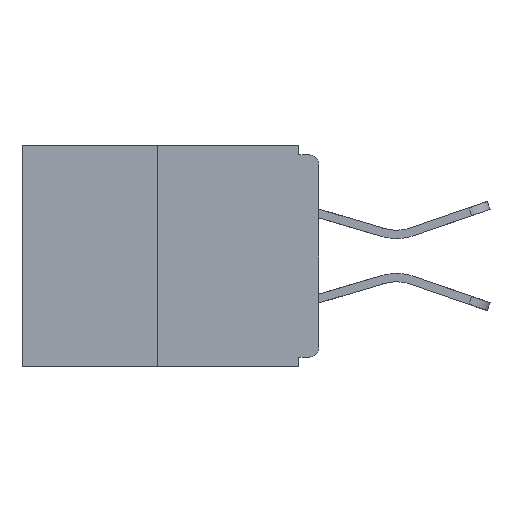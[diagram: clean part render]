
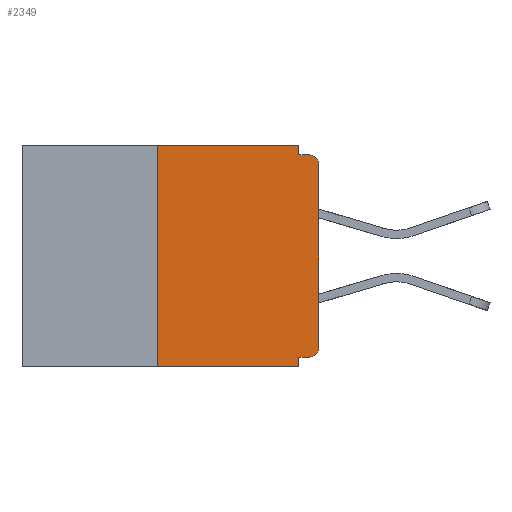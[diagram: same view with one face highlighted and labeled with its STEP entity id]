
A CAD part, left-side view. The second image highlights one B-rep face of the part: STEP entity #2349.
In plain terms, the highlighted planar face has unit normal (-1, 0, 0).
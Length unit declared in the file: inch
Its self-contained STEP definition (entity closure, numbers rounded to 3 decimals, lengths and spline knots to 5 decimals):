
#137 = VERTEX_POINT ( 'NONE', #14953 ) ;
#634 = CARTESIAN_POINT ( 'NONE',  ( 0., 0.015, -0.328 ) ) ;
#707 = DIRECTION ( 'NONE',  ( 0., -1., 0. ) ) ;
#886 = DIRECTION ( 'NONE',  ( 0., 0., -1. ) ) ;
#1024 = DIRECTION ( 'NONE',  ( 0., 0., -1. ) ) ;
#1085 = VERTEX_POINT ( 'NONE', #8054 ) ;
#1168 = PLANE ( 'NONE',  #6863 ) ;
#1349 = CARTESIAN_POINT ( 'NONE',  ( 0., 0.46, 0. ) ) ;
#1537 = AXIS2_PLACEMENT_3D ( 'NONE', #3720, #2639, #1024 ) ;
#1743 = EDGE_CURVE ( 'NONE', #15521, #137, #3775, .T. ) ;
#2099 = EDGE_CURVE ( 'NONE', #8170, #8888, #12645, .T. ) ;
#2170 = VECTOR ( 'NONE', #886, 39.37008 ) ;
#2233 = CARTESIAN_POINT ( 'NONE',  ( 0., 0., -0.015 ) ) ;
#2260 = DIRECTION ( 'NONE',  ( 0., -1., 0. ) ) ;
#2349 = ADVANCED_FACE ( 'NONE', ( #10765 ), #1168, .F. ) ;
#2639 = DIRECTION ( 'NONE',  ( -1., 0., 0. ) ) ;
#3092 = LINE ( 'NONE', #6608, #7737 ) ;
#3720 = CARTESIAN_POINT ( 'NONE',  ( 0., 0.015, -0.313 ) ) ;
#3775 = CIRCLE ( 'NONE', #1537, 0.015 ) ;
#4321 = CARTESIAN_POINT ( 'NONE',  ( 0., 0.031, 0. ) ) ;
#4432 = EDGE_CURVE ( 'NONE', #6960, #8888, #12793, .T. ) ;
#5322 = LINE ( 'NONE', #8947, #5982 ) ;
#5438 = DIRECTION ( 'NONE',  ( 0., 0., 1. ) ) ;
#5715 = LINE ( 'NONE', #12714, #10806 ) ;
#5982 = VECTOR ( 'NONE', #2260, 39.37008 ) ;
#6333 = EDGE_LOOP ( 'NONE', ( #11910, #13004, #8949, #12050, #13222, #10303, #13700, #12128, #7621, #13381 ) ) ;
#6608 = CARTESIAN_POINT ( 'NONE',  ( 0., 0., 0. ) ) ;
#6853 = CARTESIAN_POINT ( 'NONE',  ( 0., 0., -0.03 ) ) ;
#6863 = AXIS2_PLACEMENT_3D ( 'NONE', #1349, #7866, #10638 ) ;
#6960 = VERTEX_POINT ( 'NONE', #12705 ) ;
#7125 = DIRECTION ( 'NONE',  ( 0., -1., 0. ) ) ;
#7163 = DIRECTION ( 'NONE',  ( 0., 0., -1. ) ) ;
#7570 = EDGE_CURVE ( 'NONE', #1085, #13776, #5715, .T. ) ;
#7621 = ORIENTED_EDGE ( 'NONE', *, *, #4432, .F. ) ;
#7737 = VECTOR ( 'NONE', #17439, 39.37008 ) ;
#7866 = DIRECTION ( 'NONE',  ( 1., 0., 0. ) ) ;
#8054 = CARTESIAN_POINT ( 'NONE',  ( 0., 0.031, -0.328 ) ) ;
#8170 = VERTEX_POINT ( 'NONE', #6853 ) ;
#8456 = CARTESIAN_POINT ( 'NONE',  ( 0., 0.25, -0.343 ) ) ;
#8777 = VECTOR ( 'NONE', #5438, 39.37008 ) ;
#8888 = VERTEX_POINT ( 'NONE', #9609 ) ;
#8947 = CARTESIAN_POINT ( 'NONE',  ( 0., 0.46, 0. ) ) ;
#8949 = ORIENTED_EDGE ( 'NONE', *, *, #11562, .T. ) ;
#9202 = VECTOR ( 'NONE', #7125, 39.37008 ) ;
#9235 = CARTESIAN_POINT ( 'NONE',  ( 0., 0.031, -0.343 ) ) ;
#9398 = LINE ( 'NONE', #17225, #8777 ) ;
#9609 = CARTESIAN_POINT ( 'NONE',  ( 0., 0.015, -0.015 ) ) ;
#10011 = DIRECTION ( 'NONE',  ( 0., 0., -1. ) ) ;
#10303 = ORIENTED_EDGE ( 'NONE', *, *, #1743, .T. ) ;
#10353 = EDGE_CURVE ( 'NONE', #137, #8170, #3092, .T. ) ;
#10362 = CARTESIAN_POINT ( 'NONE',  ( 0., 0.031, 0. ) ) ;
#10445 = VERTEX_POINT ( 'NONE', #8456 ) ;
#10638 = DIRECTION ( 'NONE',  ( 0., 0., -1. ) ) ;
#10644 = LINE ( 'NONE', #10362, #2170 ) ;
#10765 = FACE_OUTER_BOUND ( 'NONE', #6333, .T. ) ;
#10806 = VECTOR ( 'NONE', #7163, 39.37008 ) ;
#10972 = CARTESIAN_POINT ( 'NONE',  ( 0., 0.46, -0.343 ) ) ;
#11562 = EDGE_CURVE ( 'NONE', #10445, #13776, #12371, .T. ) ;
#11846 = EDGE_CURVE ( 'NONE', #10445, #12313, #9398, .T. ) ;
#11910 = ORIENTED_EDGE ( 'NONE', *, *, #16948, .F. ) ;
#11917 = CARTESIAN_POINT ( 'NONE',  ( 0., 0.25, 0. ) ) ;
#12050 = ORIENTED_EDGE ( 'NONE', *, *, #7570, .F. ) ;
#12128 = ORIENTED_EDGE ( 'NONE', *, *, #2099, .T. ) ;
#12313 = VERTEX_POINT ( 'NONE', #11917 ) ;
#12371 = LINE ( 'NONE', #10972, #9202 ) ;
#12645 = CIRCLE ( 'NONE', #17500, 0.015 ) ;
#12705 = CARTESIAN_POINT ( 'NONE',  ( 0., 0.031, -0.015 ) ) ;
#12714 = CARTESIAN_POINT ( 'NONE',  ( 0., 0.031, -0.343 ) ) ;
#12793 = LINE ( 'NONE', #2233, #15976 ) ;
#13004 = ORIENTED_EDGE ( 'NONE', *, *, #11846, .F. ) ;
#13161 = VECTOR ( 'NONE', #15532, 39.37008 ) ;
#13222 = ORIENTED_EDGE ( 'NONE', *, *, #17331, .F. ) ;
#13381 = ORIENTED_EDGE ( 'NONE', *, *, #16916, .F. ) ;
#13700 = ORIENTED_EDGE ( 'NONE', *, *, #10353, .T. ) ;
#13776 = VERTEX_POINT ( 'NONE', #9235 ) ;
#13999 = CARTESIAN_POINT ( 'NONE',  ( 0., 0., -0.328 ) ) ;
#14399 = VERTEX_POINT ( 'NONE', #4321 ) ;
#14953 = CARTESIAN_POINT ( 'NONE',  ( 0., 0., -0.313 ) ) ;
#15521 = VERTEX_POINT ( 'NONE', #634 ) ;
#15532 = DIRECTION ( 'NONE',  ( 0., 1., 0. ) ) ;
#15916 = LINE ( 'NONE', #13999, #13161 ) ;
#15976 = VECTOR ( 'NONE', #707, 39.37008 ) ;
#16631 = CARTESIAN_POINT ( 'NONE',  ( 0., 0.015, -0.03 ) ) ;
#16695 = DIRECTION ( 'NONE',  ( -1., 0., 0. ) ) ;
#16916 = EDGE_CURVE ( 'NONE', #14399, #6960, #10644, .T. ) ;
#16948 = EDGE_CURVE ( 'NONE', #12313, #14399, #5322, .T. ) ;
#17225 = CARTESIAN_POINT ( 'NONE',  ( 0., 0.25, 0. ) ) ;
#17331 = EDGE_CURVE ( 'NONE', #15521, #1085, #15916, .T. ) ;
#17439 = DIRECTION ( 'NONE',  ( 0., 0., 1. ) ) ;
#17500 = AXIS2_PLACEMENT_3D ( 'NONE', #16631, #16695, #10011 ) ;
